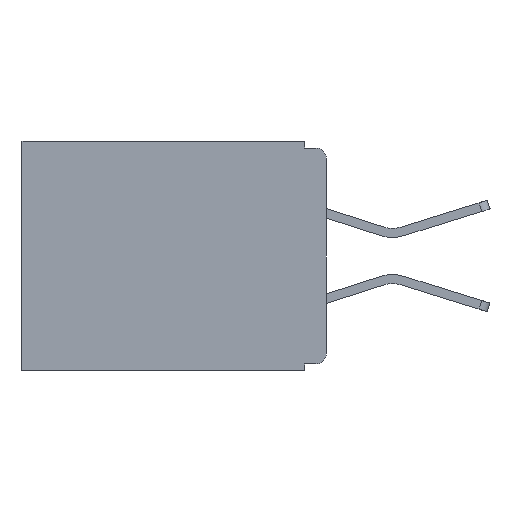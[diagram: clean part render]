
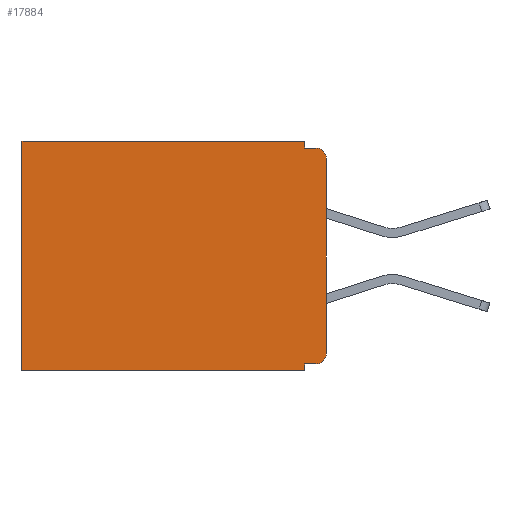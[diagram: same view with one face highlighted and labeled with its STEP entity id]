
A CAD part, left-side view. The second image highlights one B-rep face of the part: STEP entity #17884.
In plain terms, the highlighted planar face has unit normal (-1, 0, 0).
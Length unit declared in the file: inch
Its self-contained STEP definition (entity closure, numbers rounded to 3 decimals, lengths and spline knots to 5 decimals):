
#110 = VECTOR ( 'NONE', #9786, 39.37008 ) ;
#168 = EDGE_CURVE ( 'NONE', #19510, #10085, #4105, .T. ) ;
#388 = ORIENTED_EDGE ( 'NONE', *, *, #17423, .T. ) ;
#429 = VECTOR ( 'NONE', #1089, 39.37008 ) ;
#654 = CARTESIAN_POINT ( 'NONE',  ( 0.3, 0.031, -0.33 ) ) ;
#830 = DIRECTION ( 'NONE',  ( 0., 1., 0. ) ) ;
#923 = DIRECTION ( 'NONE',  ( 0., 0., -1. ) ) ;
#978 = CARTESIAN_POINT ( 'NONE',  ( 0.3, 0.031, 0. ) ) ;
#983 = LINE ( 'NONE', #21052, #429 ) ;
#1034 = EDGE_CURVE ( 'NONE', #12941, #4426, #10745, .T. ) ;
#1089 = DIRECTION ( 'NONE',  ( 0., 1., 0. ) ) ;
#1173 = ORIENTED_EDGE ( 'NONE', *, *, #17262, .T. ) ;
#1286 = DIRECTION ( 'NONE',  ( 1., 0., 0. ) ) ;
#1292 = ORIENTED_EDGE ( 'NONE', *, *, #14922, .F. ) ;
#1519 = CARTESIAN_POINT ( 'NONE',  ( 0.3, 0.015, -0.305 ) ) ;
#1597 = CARTESIAN_POINT ( 'NONE',  ( 0.3, 0., -0.01 ) ) ;
#1641 = LINE ( 'NONE', #1597, #13953 ) ;
#1778 = CARTESIAN_POINT ( 'NONE',  ( 0.3, 0.031, -0.01 ) ) ;
#2016 = CARTESIAN_POINT ( 'NONE',  ( 0.3, 0.437, -0.33 ) ) ;
#2062 = CARTESIAN_POINT ( 'NONE',  ( 0.3, 0.437, -0.33 ) ) ;
#2195 = CARTESIAN_POINT ( 'NONE',  ( 0.3, 0., -0.32 ) ) ;
#2509 = CARTESIAN_POINT ( 'NONE',  ( 0.3, 0.437, 0. ) ) ;
#2788 = ORIENTED_EDGE ( 'NONE', *, *, #5749, .F. ) ;
#3189 = DIRECTION ( 'NONE',  ( 0., 0., -1. ) ) ;
#3606 = VECTOR ( 'NONE', #830, 39.37008 ) ;
#4105 = LINE ( 'NONE', #2195, #3606 ) ;
#4230 = VERTEX_POINT ( 'NONE', #2509 ) ;
#4426 = VERTEX_POINT ( 'NONE', #2016 ) ;
#5109 = ORIENTED_EDGE ( 'NONE', *, *, #1034, .F. ) ;
#5603 = FACE_OUTER_BOUND ( 'NONE', #15529, .T. ) ;
#5717 = ORIENTED_EDGE ( 'NONE', *, *, #16028, .F. ) ;
#5749 = EDGE_CURVE ( 'NONE', #14712, #18318, #1641, .T. ) ;
#6236 = ORIENTED_EDGE ( 'NONE', *, *, #168, .F. ) ;
#6903 = VECTOR ( 'NONE', #14064, 39.37008 ) ;
#7049 = DIRECTION ( 'NONE',  ( 0., 0., -1. ) ) ;
#7076 = ORIENTED_EDGE ( 'NONE', *, *, #12351, .T. ) ;
#7448 = VERTEX_POINT ( 'NONE', #19296 ) ;
#7868 = LINE ( 'NONE', #18197, #11399 ) ;
#7892 = CARTESIAN_POINT ( 'NONE',  ( 0.3, 0., -0.33 ) ) ;
#9006 = LINE ( 'NONE', #21380, #110 ) ;
#9786 = DIRECTION ( 'NONE',  ( 0., 0., -1. ) ) ;
#10085 = VERTEX_POINT ( 'NONE', #20612 ) ;
#10745 = LINE ( 'NONE', #10889, #19049 ) ;
#10889 = CARTESIAN_POINT ( 'NONE',  ( 0.3, 0., -0.33 ) ) ;
#11023 = DIRECTION ( 'NONE',  ( -1., 0., 0. ) ) ;
#11049 = DIRECTION ( 'NONE',  ( 0., 1., 0. ) ) ;
#11388 = PLANE ( 'NONE',  #13412 ) ;
#11399 = VECTOR ( 'NONE', #19811, 39.37008 ) ;
#11492 = EDGE_CURVE ( 'NONE', #7448, #19319, #7868, .T. ) ;
#12050 = AXIS2_PLACEMENT_3D ( 'NONE', #20893, #11023, #923 ) ;
#12279 = CARTESIAN_POINT ( 'NONE',  ( 0.3, 0.031, -0.33 ) ) ;
#12351 = EDGE_CURVE ( 'NONE', #4230, #4426, #19661, .T. ) ;
#12363 = CARTESIAN_POINT ( 'NONE',  ( 0.3, 0.015, -0.01 ) ) ;
#12941 = VERTEX_POINT ( 'NONE', #12279 ) ;
#13028 = DIRECTION ( 'NONE',  ( 0., 0., -1. ) ) ;
#13261 = DIRECTION ( 'NONE',  ( -1., 0., 0. ) ) ;
#13412 = AXIS2_PLACEMENT_3D ( 'NONE', #7892, #1286, #13028 ) ;
#13953 = VECTOR ( 'NONE', #21499, 39.37008 ) ;
#14064 = DIRECTION ( 'NONE',  ( 0., 0., -1. ) ) ;
#14593 = CIRCLE ( 'NONE', #15341, 0.015 ) ;
#14697 = VECTOR ( 'NONE', #7049, 39.37008 ) ;
#14712 = VERTEX_POINT ( 'NONE', #1778 ) ;
#14922 = EDGE_CURVE ( 'NONE', #10085, #12941, #15860, .T. ) ;
#15341 = AXIS2_PLACEMENT_3D ( 'NONE', #1519, #13261, #3189 ) ;
#15529 = EDGE_LOOP ( 'NONE', ( #19562, #20887, #2788, #5717, #1173, #7076, #5109, #1292, #6236, #388 ) ) ;
#15860 = LINE ( 'NONE', #654, #6903 ) ;
#16028 = EDGE_CURVE ( 'NONE', #18472, #14712, #9006, .T. ) ;
#17262 = EDGE_CURVE ( 'NONE', #18472, #4230, #983, .T. ) ;
#17423 = EDGE_CURVE ( 'NONE', #19510, #19319, #14593, .T. ) ;
#17884 = ADVANCED_FACE ( 'NONE', ( #5603 ), #11388, .F. ) ;
#18197 = CARTESIAN_POINT ( 'NONE',  ( 0.3, 0., -0.33 ) ) ;
#18278 = CARTESIAN_POINT ( 'NONE',  ( 0.3, 0., -0.305 ) ) ;
#18318 = VERTEX_POINT ( 'NONE', #12363 ) ;
#18472 = VERTEX_POINT ( 'NONE', #978 ) ;
#19049 = VECTOR ( 'NONE', #11049, 39.37008 ) ;
#19296 = CARTESIAN_POINT ( 'NONE',  ( 0.3, 0., -0.025 ) ) ;
#19319 = VERTEX_POINT ( 'NONE', #18278 ) ;
#19510 = VERTEX_POINT ( 'NONE', #20432 ) ;
#19562 = ORIENTED_EDGE ( 'NONE', *, *, #11492, .F. ) ;
#19661 = LINE ( 'NONE', #2062, #14697 ) ;
#19690 = EDGE_CURVE ( 'NONE', #7448, #18318, #20472, .T. ) ;
#19811 = DIRECTION ( 'NONE',  ( 0., 0., -1. ) ) ;
#20432 = CARTESIAN_POINT ( 'NONE',  ( 0.3, 0.015, -0.32 ) ) ;
#20472 = CIRCLE ( 'NONE', #12050, 0.015 ) ;
#20612 = CARTESIAN_POINT ( 'NONE',  ( 0.3, 0.031, -0.32 ) ) ;
#20887 = ORIENTED_EDGE ( 'NONE', *, *, #19690, .T. ) ;
#20893 = CARTESIAN_POINT ( 'NONE',  ( 0.3, 0.015, -0.025 ) ) ;
#21052 = CARTESIAN_POINT ( 'NONE',  ( 0.3, 0., 0. ) ) ;
#21380 = CARTESIAN_POINT ( 'NONE',  ( 0.3, 0.031, 0. ) ) ;
#21499 = DIRECTION ( 'NONE',  ( 0., -1., 0. ) ) ;
